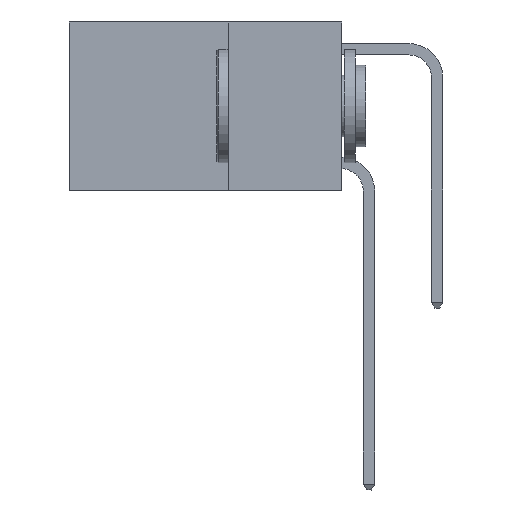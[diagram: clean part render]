
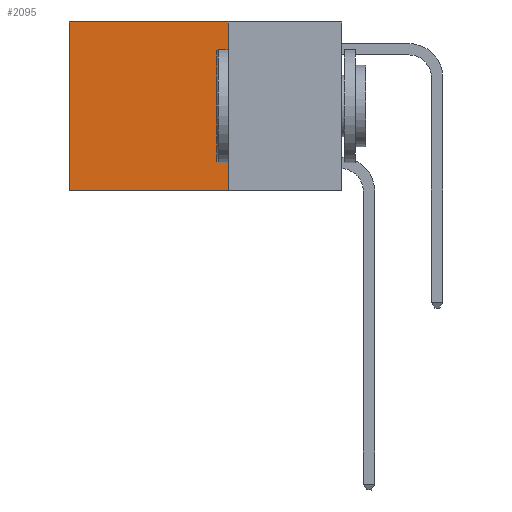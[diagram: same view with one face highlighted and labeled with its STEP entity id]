
A CAD part, left-side view. The second image highlights one B-rep face of the part: STEP entity #2095.
In plain terms, the highlighted planar face has unit normal (-1, 0, 0).
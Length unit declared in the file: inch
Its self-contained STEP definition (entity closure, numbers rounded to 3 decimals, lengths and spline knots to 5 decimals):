
#136 = DIRECTION ( 'NONE',  ( 0., 1., 0. ) ) ;
#196 = ORIENTED_EDGE ( 'NONE', *, *, #4259, .T. ) ;
#453 = EDGE_CURVE ( 'NONE', #7752, #5519, #11318, .T. ) ;
#457 = LINE ( 'NONE', #12870, #2320 ) ;
#851 = ORIENTED_EDGE ( 'NONE', *, *, #9430, .F. ) ;
#894 = DIRECTION ( 'NONE',  ( 1., 0., 0. ) ) ;
#955 = CARTESIAN_POINT ( 'NONE',  ( 0.2625, 0.6, -0.37 ) ) ;
#1122 = EDGE_CURVE ( 'NONE', #8177, #4426, #457, .T. ) ;
#2095 = ADVANCED_FACE ( 'NONE', ( #6889 ), #10983, .F. ) ;
#2195 = CARTESIAN_POINT ( 'NONE',  ( 0.2625, 0.6, 0. ) ) ;
#2320 = VECTOR ( 'NONE', #7617, 39.37008 ) ;
#3820 = EDGE_LOOP ( 'NONE', ( #11820, #851, #11773, #196 ) ) ;
#4252 = LINE ( 'NONE', #4374, #9077 ) ;
#4259 = EDGE_CURVE ( 'NONE', #8177, #7752, #4252, .T. ) ;
#4374 = CARTESIAN_POINT ( 'NONE',  ( 0.2625, 0.25, 0. ) ) ;
#4426 = VERTEX_POINT ( 'NONE', #12618 ) ;
#4473 = DIRECTION ( 'NONE',  ( 0., 1., 0. ) ) ;
#4985 = DIRECTION ( 'NONE',  ( 0., 0., -1. ) ) ;
#5519 = VERTEX_POINT ( 'NONE', #955 ) ;
#5897 = CARTESIAN_POINT ( 'NONE',  ( 0.2625, 0.25, 0. ) ) ;
#6478 = VECTOR ( 'NONE', #4473, 39.37008 ) ;
#6554 = CARTESIAN_POINT ( 'NONE',  ( 0.2625, 0.25, 0. ) ) ;
#6889 = FACE_OUTER_BOUND ( 'NONE', #3820, .T. ) ;
#7286 = DIRECTION ( 'NONE',  ( 0., 0., -1. ) ) ;
#7381 = LINE ( 'NONE', #11535, #6478 ) ;
#7617 = DIRECTION ( 'NONE',  ( 0., 0., -1. ) ) ;
#7752 = VERTEX_POINT ( 'NONE', #9214 ) ;
#8177 = VERTEX_POINT ( 'NONE', #6554 ) ;
#9077 = VECTOR ( 'NONE', #136, 39.37008 ) ;
#9134 = AXIS2_PLACEMENT_3D ( 'NONE', #5897, #894, #4985 ) ;
#9214 = CARTESIAN_POINT ( 'NONE',  ( 0.2625, 0.6, 0. ) ) ;
#9430 = EDGE_CURVE ( 'NONE', #4426, #5519, #7381, .T. ) ;
#9933 = VECTOR ( 'NONE', #7286, 39.37008 ) ;
#10983 = PLANE ( 'NONE',  #9134 ) ;
#11318 = LINE ( 'NONE', #2195, #9933 ) ;
#11535 = CARTESIAN_POINT ( 'NONE',  ( 0.2625, 0.25, -0.37 ) ) ;
#11773 = ORIENTED_EDGE ( 'NONE', *, *, #1122, .F. ) ;
#11820 = ORIENTED_EDGE ( 'NONE', *, *, #453, .T. ) ;
#12618 = CARTESIAN_POINT ( 'NONE',  ( 0.2625, 0.25, -0.37 ) ) ;
#12870 = CARTESIAN_POINT ( 'NONE',  ( 0.2625, 0.25, 0. ) ) ;
